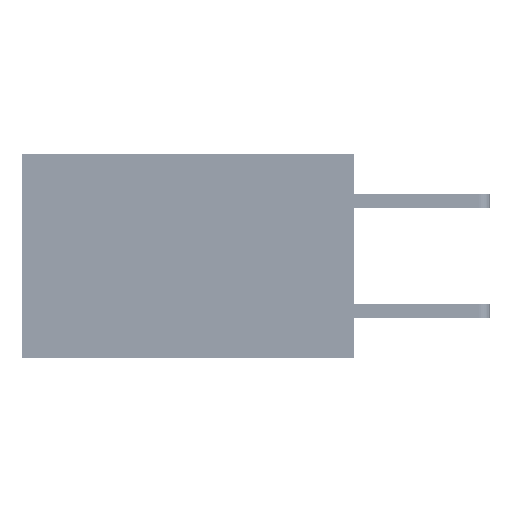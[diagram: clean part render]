
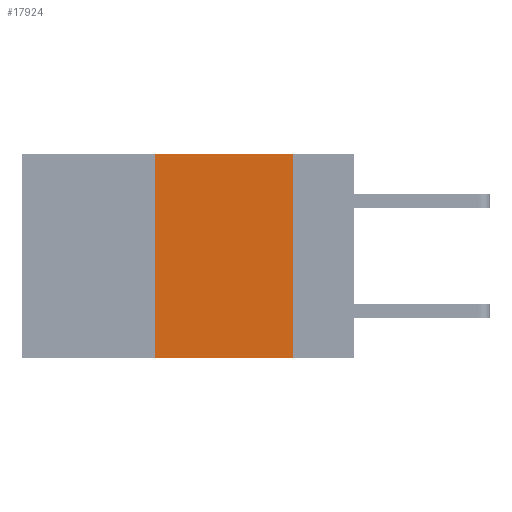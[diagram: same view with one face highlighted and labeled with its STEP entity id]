
A CAD part, left-side view. The second image highlights one B-rep face of the part: STEP entity #17924.
In plain terms, the highlighted planar face has unit normal (-1, 0, 0).
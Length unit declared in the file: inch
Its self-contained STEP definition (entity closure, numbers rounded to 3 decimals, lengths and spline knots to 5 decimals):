
#290 = CARTESIAN_POINT ( 'NONE',  ( 0., 0.6, 0. ) ) ;
#536 = FACE_OUTER_BOUND ( 'NONE', #38509, .T. ) ;
#939 = ORIENTED_EDGE ( 'NONE', *, *, #31797, .F. ) ;
#3616 = VECTOR ( 'NONE', #46155, 39.37008 ) ;
#4127 = DIRECTION ( 'NONE',  ( 0., 0., -1. ) ) ;
#4748 = ORIENTED_EDGE ( 'NONE', *, *, #31153, .F. ) ;
#5482 = VERTEX_POINT ( 'NONE', #13937 ) ;
#6352 = VERTEX_POINT ( 'NONE', #28150 ) ;
#7987 = CARTESIAN_POINT ( 'NONE',  ( 0., 0.11, 0. ) ) ;
#9618 = EDGE_CURVE ( 'NONE', #6352, #41016, #24322, .T. ) ;
#13937 = CARTESIAN_POINT ( 'NONE',  ( 0., 0.36, 0. ) ) ;
#14541 = CARTESIAN_POINT ( 'NONE',  ( 0., 0.11, 0. ) ) ;
#15058 = DIRECTION ( 'NONE',  ( 1., 0., 0. ) ) ;
#16514 = VERTEX_POINT ( 'NONE', #7987 ) ;
#17259 = CARTESIAN_POINT ( 'NONE',  ( 0., 0.11, -0.37 ) ) ;
#17924 = ADVANCED_FACE ( 'NONE', ( #536 ), #33440, .F. ) ;
#19036 = VECTOR ( 'NONE', #34932, 39.37008 ) ;
#21261 = LINE ( 'NONE', #35507, #3616 ) ;
#22578 = DIRECTION ( 'NONE',  ( 0., 0., -1. ) ) ;
#23808 = EDGE_CURVE ( 'NONE', #16514, #41016, #36297, .T. ) ;
#24322 = LINE ( 'NONE', #43134, #19036 ) ;
#24985 = AXIS2_PLACEMENT_3D ( 'NONE', #290, #15058, #22578 ) ;
#26853 = ORIENTED_EDGE ( 'NONE', *, *, #23808, .F. ) ;
#28150 = CARTESIAN_POINT ( 'NONE',  ( 0., 0.36, -0.37 ) ) ;
#31153 = EDGE_CURVE ( 'NONE', #6352, #5482, #21261, .T. ) ;
#31797 = EDGE_CURVE ( 'NONE', #5482, #16514, #38749, .T. ) ;
#33440 = PLANE ( 'NONE',  #24985 ) ;
#34040 = VECTOR ( 'NONE', #4127, 39.37008 ) ;
#34932 = DIRECTION ( 'NONE',  ( 0., -1., 0. ) ) ;
#35507 = CARTESIAN_POINT ( 'NONE',  ( 0., 0.36, 0. ) ) ;
#36297 = LINE ( 'NONE', #14541, #34040 ) ;
#37371 = ORIENTED_EDGE ( 'NONE', *, *, #9618, .T. ) ;
#38509 = EDGE_LOOP ( 'NONE', ( #26853, #939, #4748, #37371 ) ) ;
#38749 = LINE ( 'NONE', #39874, #44850 ) ;
#39874 = CARTESIAN_POINT ( 'NONE',  ( 0., 0.6, 0. ) ) ;
#41016 = VERTEX_POINT ( 'NONE', #17259 ) ;
#43134 = CARTESIAN_POINT ( 'NONE',  ( 0., 0.6, -0.37 ) ) ;
#44850 = VECTOR ( 'NONE', #45522, 39.37008 ) ;
#45522 = DIRECTION ( 'NONE',  ( 0., -1., 0. ) ) ;
#46155 = DIRECTION ( 'NONE',  ( 0., 0., 1. ) ) ;
